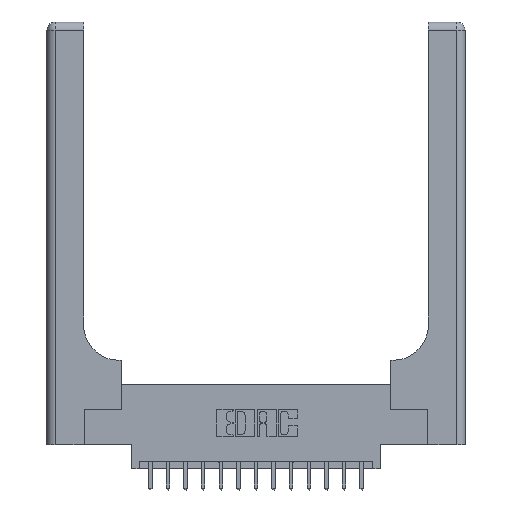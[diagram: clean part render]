
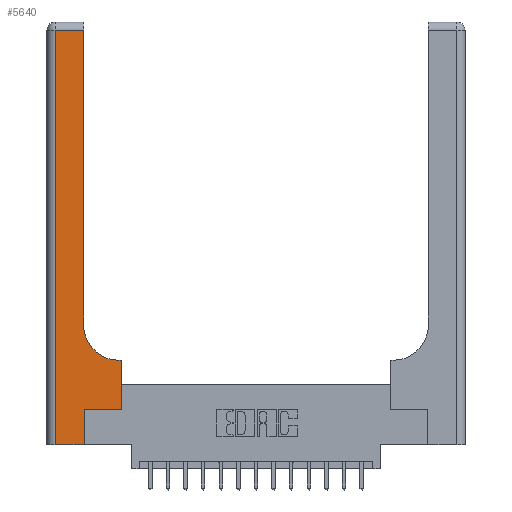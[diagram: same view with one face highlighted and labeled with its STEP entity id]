
A CAD part, top view. The second image highlights one B-rep face of the part: STEP entity #5640.
In plain terms, the highlighted planar face has unit normal (0, 0, 1).
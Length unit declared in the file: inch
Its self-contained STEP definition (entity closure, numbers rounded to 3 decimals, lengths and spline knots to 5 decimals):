
#160 = ORIENTED_EDGE ( 'NONE', *, *, #12675, .T. ) ;
#228 = LINE ( 'NONE', #4362, #9290 ) ;
#430 = VERTEX_POINT ( 'NONE', #6115 ) ;
#877 = VECTOR ( 'NONE', #4494, 39.37008 ) ;
#1102 = CARTESIAN_POINT ( 'NONE',  ( 0.26, 0.85, 0.37 ) ) ;
#1247 = EDGE_CURVE ( 'NONE', #3327, #430, #17141, .T. ) ;
#1356 = DIRECTION ( 'NONE',  ( 1., 0., 0. ) ) ;
#1571 = CARTESIAN_POINT ( 'NONE',  ( 0.06, 3., 0.37 ) ) ;
#1573 = CARTESIAN_POINT ( 'NONE',  ( 0.528, 0.25, 0.37 ) ) ;
#2159 = CARTESIAN_POINT ( 'NONE',  ( 0.06, 0., 0.37 ) ) ;
#2350 = ORIENTED_EDGE ( 'NONE', *, *, #14393, .T. ) ;
#2413 = VECTOR ( 'NONE', #4437, 39.37008 ) ;
#2951 = DIRECTION ( 'NONE',  ( 0., 1., 0. ) ) ;
#2981 = LINE ( 'NONE', #15741, #2413 ) ;
#3106 = CARTESIAN_POINT ( 'NONE',  ( 0., 0., 0.37 ) ) ;
#3292 = EDGE_CURVE ( 'NONE', #7104, #17857, #4223, .T. ) ;
#3327 = VERTEX_POINT ( 'NONE', #4850 ) ;
#4223 = LINE ( 'NONE', #1571, #877 ) ;
#4362 = CARTESIAN_POINT ( 'NONE',  ( 0.265, 0.25, 0.37 ) ) ;
#4437 = DIRECTION ( 'NONE',  ( 0., 1., 0. ) ) ;
#4494 = DIRECTION ( 'NONE',  ( 0., -1., 0. ) ) ;
#4850 = CARTESIAN_POINT ( 'NONE',  ( 0.528, 0.6, 0.37 ) ) ;
#5013 = VECTOR ( 'NONE', #8760, 39.37008 ) ;
#5487 = EDGE_CURVE ( 'NONE', #5571, #3327, #6820, .T. ) ;
#5562 = CIRCLE ( 'NONE', #15224, 0.25 ) ;
#5571 = VERTEX_POINT ( 'NONE', #13786 ) ;
#5640 = ADVANCED_FACE ( 'NONE', ( #15809 ), #7632, .F. ) ;
#6058 = ORIENTED_EDGE ( 'NONE', *, *, #1247, .T. ) ;
#6115 = CARTESIAN_POINT ( 'NONE',  ( 0.51, 0.6, 0.37 ) ) ;
#6504 = ORIENTED_EDGE ( 'NONE', *, *, #3292, .T. ) ;
#6820 = LINE ( 'NONE', #1573, #15245 ) ;
#7104 = VERTEX_POINT ( 'NONE', #17983 ) ;
#7363 = EDGE_LOOP ( 'NONE', ( #8910, #17749, #6504, #9001, #2350, #160, #16088, #6058, #8641 ) ) ;
#7390 = CARTESIAN_POINT ( 'NONE',  ( 0., 2.94, 0.37 ) ) ;
#7632 = PLANE ( 'NONE',  #8838 ) ;
#8641 = ORIENTED_EDGE ( 'NONE', *, *, #11197, .T. ) ;
#8760 = DIRECTION ( 'NONE',  ( -1., 0., 0. ) ) ;
#8838 = AXIS2_PLACEMENT_3D ( 'NONE', #13240, #13061, #14339 ) ;
#8910 = ORIENTED_EDGE ( 'NONE', *, *, #17517, .T. ) ;
#9001 = ORIENTED_EDGE ( 'NONE', *, *, #15148, .T. ) ;
#9290 = VECTOR ( 'NONE', #11620, 39.37008 ) ;
#10133 = LINE ( 'NONE', #7390, #5013 ) ;
#10178 = VECTOR ( 'NONE', #10616, 39.37008 ) ;
#10559 = VERTEX_POINT ( 'NONE', #14728 ) ;
#10564 = VERTEX_POINT ( 'NONE', #14547 ) ;
#10616 = DIRECTION ( 'NONE',  ( 0., 1., 0. ) ) ;
#11197 = EDGE_CURVE ( 'NONE', #430, #13424, #5562, .T. ) ;
#11353 = DIRECTION ( 'NONE',  ( -1., 0., 0. ) ) ;
#11392 = LINE ( 'NONE', #3106, #15372 ) ;
#11620 = DIRECTION ( 'NONE',  ( 1., 0., 0. ) ) ;
#12128 = EDGE_CURVE ( 'NONE', #10559, #7104, #10133, .T. ) ;
#12161 = CARTESIAN_POINT ( 'NONE',  ( 0.265, 0., 0.37 ) ) ;
#12214 = DIRECTION ( 'NONE',  ( 0., 0., -1. ) ) ;
#12675 = EDGE_CURVE ( 'NONE', #10564, #5571, #228, .T. ) ;
#13061 = DIRECTION ( 'NONE',  ( 0., 0., -1. ) ) ;
#13240 = CARTESIAN_POINT ( 'NONE',  ( 0., 3., 0.37 ) ) ;
#13424 = VERTEX_POINT ( 'NONE', #1102 ) ;
#13786 = CARTESIAN_POINT ( 'NONE',  ( 0.528, 0.25, 0.37 ) ) ;
#14069 = VERTEX_POINT ( 'NONE', #12161 ) ;
#14339 = DIRECTION ( 'NONE',  ( -1., 0., 0. ) ) ;
#14393 = EDGE_CURVE ( 'NONE', #14069, #10564, #2981, .T. ) ;
#14547 = CARTESIAN_POINT ( 'NONE',  ( 0.265, 0.25, 0.37 ) ) ;
#14728 = CARTESIAN_POINT ( 'NONE',  ( 0.26, 2.94, 0.37 ) ) ;
#15148 = EDGE_CURVE ( 'NONE', #17857, #14069, #11392, .T. ) ;
#15224 = AXIS2_PLACEMENT_3D ( 'NONE', #17994, #12214, #17813 ) ;
#15245 = VECTOR ( 'NONE', #2951, 39.37008 ) ;
#15372 = VECTOR ( 'NONE', #1356, 39.37008 ) ;
#15741 = CARTESIAN_POINT ( 'NONE',  ( 0.265, 0., 0.37 ) ) ;
#15809 = FACE_OUTER_BOUND ( 'NONE', #7363, .T. ) ;
#16088 = ORIENTED_EDGE ( 'NONE', *, *, #5487, .T. ) ;
#17052 = CARTESIAN_POINT ( 'NONE',  ( 0.26, 0.6, 0.37 ) ) ;
#17141 = LINE ( 'NONE', #17052, #17181 ) ;
#17181 = VECTOR ( 'NONE', #11353, 39.37008 ) ;
#17426 = CARTESIAN_POINT ( 'NONE',  ( 0.26, 3., 0.37 ) ) ;
#17517 = EDGE_CURVE ( 'NONE', #13424, #10559, #17595, .T. ) ;
#17595 = LINE ( 'NONE', #17426, #10178 ) ;
#17749 = ORIENTED_EDGE ( 'NONE', *, *, #12128, .T. ) ;
#17813 = DIRECTION ( 'NONE',  ( 1., 0., 0. ) ) ;
#17857 = VERTEX_POINT ( 'NONE', #2159 ) ;
#17983 = CARTESIAN_POINT ( 'NONE',  ( 0.06, 2.94, 0.37 ) ) ;
#17994 = CARTESIAN_POINT ( 'NONE',  ( 0.51, 0.85, 0.37 ) ) ;
